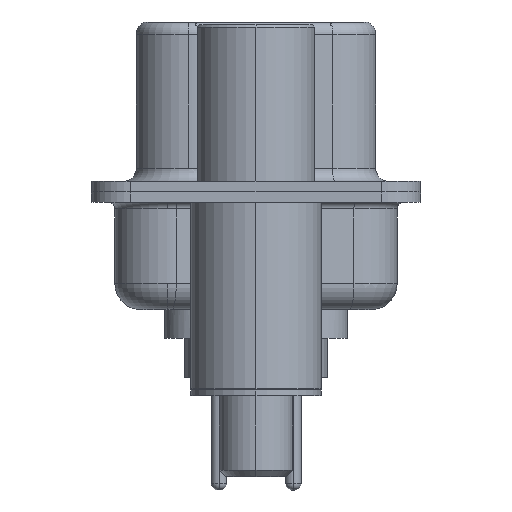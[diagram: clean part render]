
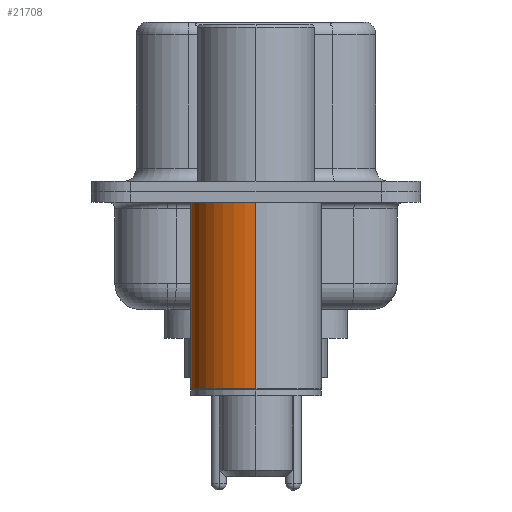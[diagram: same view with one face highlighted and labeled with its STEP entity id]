
A CAD part, left-side view. The second image highlights one B-rep face of the part: STEP entity #21708.
In plain terms, the highlighted cylindrical face has radius 2.5 mm (diameter 5 mm), a partial arc.
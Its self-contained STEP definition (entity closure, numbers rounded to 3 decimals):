
#953 = CYLINDRICAL_SURFACE ( 'NONE', #16173, 2.5 ) ;
#2258 = DIRECTION ( 'NONE',  ( 1., 0., 0. ) ) ;
#2868 = ORIENTED_EDGE ( 'NONE', *, *, #10461, .T. ) ;
#2953 = EDGE_CURVE ( 'NONE', #22774, #20760, #4788, .T. ) ;
#4041 = VECTOR ( 'NONE', #24191, 1000. ) ;
#4788 = LINE ( 'NONE', #18071, #4041 ) ;
#4906 = CIRCLE ( 'NONE', #18626, 2.5 ) ;
#6146 = CARTESIAN_POINT ( 'NONE',  ( 2.5, 0., 0.581 ) ) ;
#6861 = CARTESIAN_POINT ( 'NONE',  ( -2.5, 0., -7.525 ) ) ;
#6948 = DIRECTION ( 'NONE',  ( 0., 0., 1. ) ) ;
#7041 = CARTESIAN_POINT ( 'NONE',  ( 2.5, 0., -7.525 ) ) ;
#7622 = ORIENTED_EDGE ( 'NONE', *, *, #24159, .F. ) ;
#8274 = LINE ( 'NONE', #6146, #24968 ) ;
#9541 = DIRECTION ( 'NONE',  ( 0., 0., 1. ) ) ;
#10461 = EDGE_CURVE ( 'NONE', #25354, #22774, #4906, .T. ) ;
#10561 = DIRECTION ( 'NONE',  ( 0., 0., 1. ) ) ;
#11717 = DIRECTION ( 'NONE',  ( 1., 0., 0. ) ) ;
#13628 = VERTEX_POINT ( 'NONE', #14683 ) ;
#14683 = CARTESIAN_POINT ( 'NONE',  ( 2.5, 0., -0.4 ) ) ;
#15626 = DIRECTION ( 'NONE',  ( 0., 0., 1. ) ) ;
#15663 = AXIS2_PLACEMENT_3D ( 'NONE', #20046, #6948, #22206 ) ;
#16173 = AXIS2_PLACEMENT_3D ( 'NONE', #18380, #9541, #11717 ) ;
#16918 = EDGE_CURVE ( 'NONE', #25354, #13628, #8274, .T. ) ;
#17649 = CIRCLE ( 'NONE', #15663, 2.5 ) ;
#18071 = CARTESIAN_POINT ( 'NONE',  ( -2.5, 0., 0.581 ) ) ;
#18318 = EDGE_LOOP ( 'NONE', ( #2868, #19008, #7622, #24032 ) ) ;
#18380 = CARTESIAN_POINT ( 'NONE',  ( 0., 0., 0.581 ) ) ;
#18626 = AXIS2_PLACEMENT_3D ( 'NONE', #28598, #15626, #2258 ) ;
#18744 = FACE_OUTER_BOUND ( 'NONE', #18318, .T. ) ;
#19008 = ORIENTED_EDGE ( 'NONE', *, *, #2953, .T. ) ;
#20046 = CARTESIAN_POINT ( 'NONE',  ( 0., 0., -0.4 ) ) ;
#20760 = VERTEX_POINT ( 'NONE', #24782 ) ;
#21708 = ADVANCED_FACE ( 'NONE', ( #18744 ), #953, .T. ) ;
#22206 = DIRECTION ( 'NONE',  ( 1., 0., 0. ) ) ;
#22774 = VERTEX_POINT ( 'NONE', #6861 ) ;
#24032 = ORIENTED_EDGE ( 'NONE', *, *, #16918, .F. ) ;
#24159 = EDGE_CURVE ( 'NONE', #13628, #20760, #17649, .T. ) ;
#24191 = DIRECTION ( 'NONE',  ( 0., 0., 1. ) ) ;
#24782 = CARTESIAN_POINT ( 'NONE',  ( -2.5, 0., -0.4 ) ) ;
#24968 = VECTOR ( 'NONE', #10561, 1000. ) ;
#25354 = VERTEX_POINT ( 'NONE', #7041 ) ;
#28598 = CARTESIAN_POINT ( 'NONE',  ( 0., 0., -7.525 ) ) ;
